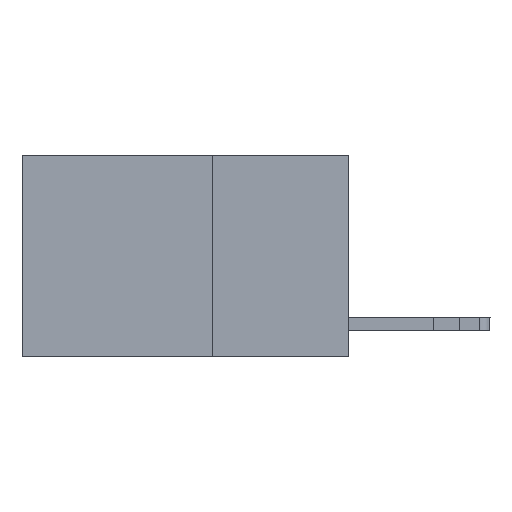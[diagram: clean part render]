
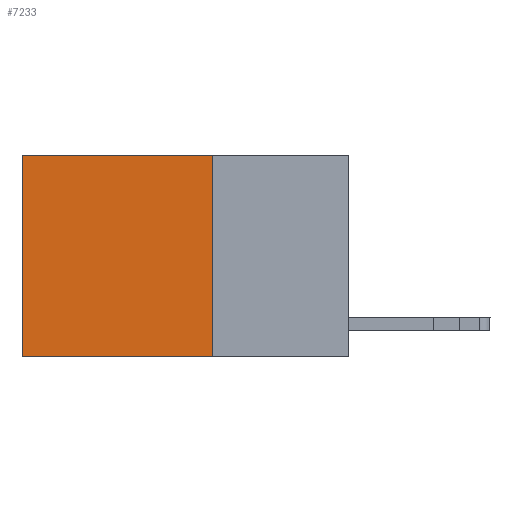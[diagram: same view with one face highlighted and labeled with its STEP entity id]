
A CAD part, left-side view. The second image highlights one B-rep face of the part: STEP entity #7233.
In plain terms, the highlighted planar face has unit normal (-1, 0, 0).
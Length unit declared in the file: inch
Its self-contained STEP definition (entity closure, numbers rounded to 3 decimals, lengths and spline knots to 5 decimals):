
#77 = VECTOR ( 'NONE', #5548, 39.37008 ) ;
#1333 = PLANE ( 'NONE',  #11309 ) ;
#2039 = DIRECTION ( 'NONE',  ( 0., 0., -1. ) ) ;
#3145 = ORIENTED_EDGE ( 'NONE', *, *, #8578, .F. ) ;
#3226 = VERTEX_POINT ( 'NONE', #16645 ) ;
#3306 = CARTESIAN_POINT ( 'NONE',  ( 0.2625, 0.25, 0. ) ) ;
#3630 = CARTESIAN_POINT ( 'NONE',  ( 0.2625, 0.6, 0. ) ) ;
#3869 = VECTOR ( 'NONE', #15406, 39.37008 ) ;
#4086 = CARTESIAN_POINT ( 'NONE',  ( 0.2625, 0.6, 0. ) ) ;
#5059 = ORIENTED_EDGE ( 'NONE', *, *, #10727, .T. ) ;
#5081 = CARTESIAN_POINT ( 'NONE',  ( 0.2625, 0.25, -0.37 ) ) ;
#5548 = DIRECTION ( 'NONE',  ( 0., 1., 0. ) ) ;
#5892 = CARTESIAN_POINT ( 'NONE',  ( 0.2625, 0.25, 0. ) ) ;
#6178 = EDGE_CURVE ( 'NONE', #3226, #12222, #16277, .T. ) ;
#6221 = VECTOR ( 'NONE', #2039, 39.37008 ) ;
#6297 = LINE ( 'NONE', #3306, #3869 ) ;
#6850 = LINE ( 'NONE', #14462, #15906 ) ;
#7233 = ADVANCED_FACE ( 'NONE', ( #11746 ), #1333, .F. ) ;
#8578 = EDGE_CURVE ( 'NONE', #14207, #3226, #6297, .T. ) ;
#10575 = ORIENTED_EDGE ( 'NONE', *, *, #18609, .T. ) ;
#10727 = EDGE_CURVE ( 'NONE', #11806, #12222, #14141, .T. ) ;
#11083 = CARTESIAN_POINT ( 'NONE',  ( 0.2625, 0.25, 0. ) ) ;
#11309 = AXIS2_PLACEMENT_3D ( 'NONE', #5892, #13338, #16613 ) ;
#11746 = FACE_OUTER_BOUND ( 'NONE', #12140, .T. ) ;
#11806 = VERTEX_POINT ( 'NONE', #4086 ) ;
#12140 = EDGE_LOOP ( 'NONE', ( #5059, #13464, #3145, #10575 ) ) ;
#12222 = VERTEX_POINT ( 'NONE', #18974 ) ;
#12876 = DIRECTION ( 'NONE',  ( 0., 1., 0. ) ) ;
#13338 = DIRECTION ( 'NONE',  ( 1., 0., 0. ) ) ;
#13464 = ORIENTED_EDGE ( 'NONE', *, *, #6178, .F. ) ;
#14141 = LINE ( 'NONE', #3630, #6221 ) ;
#14207 = VERTEX_POINT ( 'NONE', #11083 ) ;
#14462 = CARTESIAN_POINT ( 'NONE',  ( 0.2625, 0.25, 0. ) ) ;
#15406 = DIRECTION ( 'NONE',  ( 0., 0., -1. ) ) ;
#15906 = VECTOR ( 'NONE', #12876, 39.37008 ) ;
#16277 = LINE ( 'NONE', #5081, #77 ) ;
#16613 = DIRECTION ( 'NONE',  ( 0., 0., -1. ) ) ;
#16645 = CARTESIAN_POINT ( 'NONE',  ( 0.2625, 0.25, -0.37 ) ) ;
#18609 = EDGE_CURVE ( 'NONE', #14207, #11806, #6850, .T. ) ;
#18974 = CARTESIAN_POINT ( 'NONE',  ( 0.2625, 0.6, -0.37 ) ) ;
